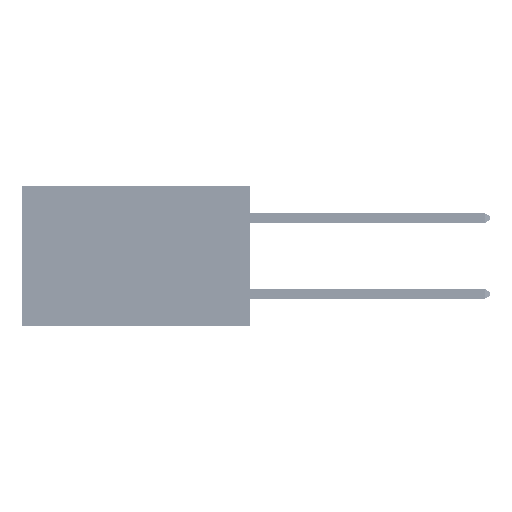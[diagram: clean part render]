
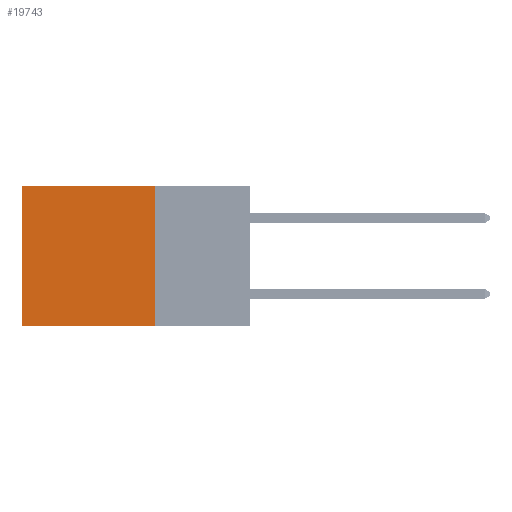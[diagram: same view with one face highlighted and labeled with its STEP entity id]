
A CAD part, left-side view. The second image highlights one B-rep face of the part: STEP entity #19743.
In plain terms, the highlighted planar face has unit normal (-1, 0, 0).
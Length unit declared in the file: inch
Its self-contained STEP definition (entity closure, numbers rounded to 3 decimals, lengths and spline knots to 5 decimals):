
#69 = CARTESIAN_POINT ( 'NONE',  ( 0.2875, 0.25, 0. ) ) ;
#9677 = CARTESIAN_POINT ( 'NONE',  ( 0.2875, 0.25, -0.37 ) ) ;
#10959 = EDGE_CURVE ( 'NONE', #17024, #11171, #15621, .T. ) ;
#11171 = VERTEX_POINT ( 'NONE', #9677 ) ;
#11915 = VECTOR ( 'NONE', #22477, 39.37008 ) ;
#12612 = CARTESIAN_POINT ( 'NONE',  ( 0.2875, 0.6, 0. ) ) ;
#12634 = DIRECTION ( 'NONE',  ( 0., 0., -1. ) ) ;
#12949 = VECTOR ( 'NONE', #28120, 39.37008 ) ;
#15621 = LINE ( 'NONE', #24767, #18742 ) ;
#16598 = AXIS2_PLACEMENT_3D ( 'NONE', #33780, #42065, #18345 ) ;
#16608 = EDGE_CURVE ( 'NONE', #11171, #44784, #31750, .T. ) ;
#17024 = VERTEX_POINT ( 'NONE', #28737 ) ;
#17025 = VERTEX_POINT ( 'NONE', #12612 ) ;
#17998 = PLANE ( 'NONE',  #16598 ) ;
#18345 = DIRECTION ( 'NONE',  ( 0., 0., -1. ) ) ;
#18742 = VECTOR ( 'NONE', #12634, 39.37008 ) ;
#19743 = ADVANCED_FACE ( 'NONE', ( #37514 ), #17998, .F. ) ;
#21484 = ORIENTED_EDGE ( 'NONE', *, *, #21888, .T. ) ;
#21888 = EDGE_CURVE ( 'NONE', #17025, #44784, #31707, .T. ) ;
#22477 = DIRECTION ( 'NONE',  ( 0., 1., 0. ) ) ;
#24767 = CARTESIAN_POINT ( 'NONE',  ( 0.2875, 0.25, 0. ) ) ;
#25952 = CARTESIAN_POINT ( 'NONE',  ( 0.2875, 0.6, 0. ) ) ;
#26452 = CARTESIAN_POINT ( 'NONE',  ( 0.2875, 0.25, -0.37 ) ) ;
#28120 = DIRECTION ( 'NONE',  ( 0., 1., 0. ) ) ;
#28385 = CARTESIAN_POINT ( 'NONE',  ( 0.2875, 0.6, -0.37 ) ) ;
#28737 = CARTESIAN_POINT ( 'NONE',  ( 0.2875, 0.25, 0. ) ) ;
#31673 = ORIENTED_EDGE ( 'NONE', *, *, #16608, .F. ) ;
#31707 = LINE ( 'NONE', #25952, #37270 ) ;
#31750 = LINE ( 'NONE', #26452, #11915 ) ;
#33780 = CARTESIAN_POINT ( 'NONE',  ( 0.2875, 0.25, 0. ) ) ;
#34227 = ORIENTED_EDGE ( 'NONE', *, *, #49705, .T. ) ;
#37270 = VECTOR ( 'NONE', #42183, 39.37008 ) ;
#37514 = FACE_OUTER_BOUND ( 'NONE', #50843, .T. ) ;
#42065 = DIRECTION ( 'NONE',  ( 1., 0., 0. ) ) ;
#42183 = DIRECTION ( 'NONE',  ( 0., 0., -1. ) ) ;
#44784 = VERTEX_POINT ( 'NONE', #28385 ) ;
#49705 = EDGE_CURVE ( 'NONE', #17024, #17025, #49985, .T. ) ;
#49985 = LINE ( 'NONE', #69, #12949 ) ;
#50843 = EDGE_LOOP ( 'NONE', ( #21484, #31673, #50938, #34227 ) ) ;
#50938 = ORIENTED_EDGE ( 'NONE', *, *, #10959, .F. ) ;
